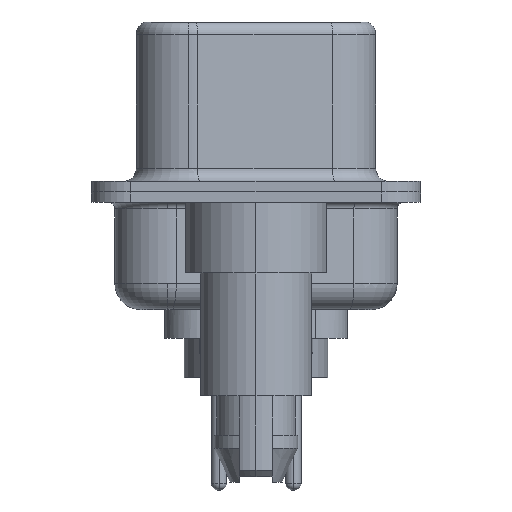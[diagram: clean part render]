
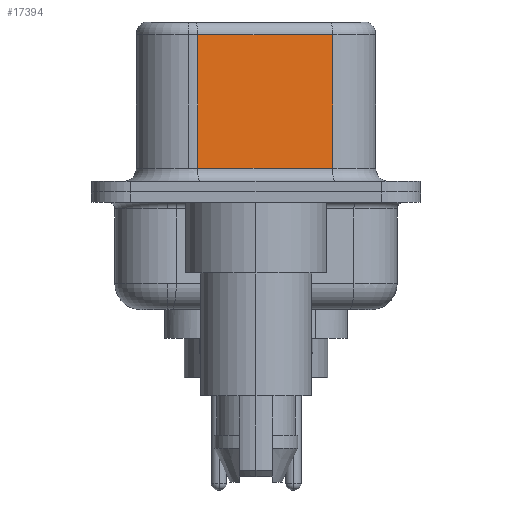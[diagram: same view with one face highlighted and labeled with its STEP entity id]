
A CAD part, left-side view. The second image highlights one B-rep face of the part: STEP entity #17394.
In plain terms, the highlighted planar face has unit normal (-0.985, -0.174, 0).
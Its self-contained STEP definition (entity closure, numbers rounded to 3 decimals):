
#341 = EDGE_CURVE ( 'NONE', #7643, #17818, #17907, .T. ) ;
#493 = EDGE_LOOP ( 'NONE', ( #12141, #4127, #10925, #8058 ) ) ;
#1292 = VERTEX_POINT ( 'NONE', #5120 ) ;
#1805 = CARTESIAN_POINT ( 'NONE',  ( 3.67, 2.233, 6.52 ) ) ;
#2773 = CARTESIAN_POINT ( 'NONE',  ( 4.58, -2.927, 0.9 ) ) ;
#2933 = VECTOR ( 'NONE', #13333, 1000. ) ;
#3874 = DIRECTION ( 'NONE',  ( 0.985, 0.174, 0. ) ) ;
#4127 = ORIENTED_EDGE ( 'NONE', *, *, #16135, .T. ) ;
#5120 = CARTESIAN_POINT ( 'NONE',  ( 4.58, -2.927, 6.02 ) ) ;
#5962 = VECTOR ( 'NONE', #15176, 1000. ) ;
#6122 = LINE ( 'NONE', #9501, #17211 ) ;
#7643 = VERTEX_POINT ( 'NONE', #9998 ) ;
#7668 = DIRECTION ( 'NONE',  ( 0.174, -0.985, 0. ) ) ;
#8058 = ORIENTED_EDGE ( 'NONE', *, *, #9245, .T. ) ;
#9245 = EDGE_CURVE ( 'NONE', #17818, #10702, #14181, .T. ) ;
#9501 = CARTESIAN_POINT ( 'NONE',  ( 4.58, -2.927, 6.52 ) ) ;
#9619 = PLANE ( 'NONE',  #16470 ) ;
#9998 = CARTESIAN_POINT ( 'NONE',  ( 3.67, 2.233, 6.02 ) ) ;
#10250 = LINE ( 'NONE', #17977, #5962 ) ;
#10702 = VERTEX_POINT ( 'NONE', #2773 ) ;
#10704 = VECTOR ( 'NONE', #7668, 1000. ) ;
#10925 = ORIENTED_EDGE ( 'NONE', *, *, #341, .T. ) ;
#11237 = EDGE_CURVE ( 'NONE', #1292, #10702, #6122, .T. ) ;
#12141 = ORIENTED_EDGE ( 'NONE', *, *, #11237, .F. ) ;
#12255 = CARTESIAN_POINT ( 'NONE',  ( 3.67, 2.233, 0.9 ) ) ;
#12589 = CARTESIAN_POINT ( 'NONE',  ( 4.58, -2.927, 6.52 ) ) ;
#13333 = DIRECTION ( 'NONE',  ( 0., 0., -1. ) ) ;
#14100 = DIRECTION ( 'NONE',  ( -0.174, 0.985, 0. ) ) ;
#14181 = LINE ( 'NONE', #17807, #10704 ) ;
#15176 = DIRECTION ( 'NONE',  ( -0.174, 0.985, 0. ) ) ;
#16135 = EDGE_CURVE ( 'NONE', #1292, #7643, #10250, .T. ) ;
#16470 = AXIS2_PLACEMENT_3D ( 'NONE', #12589, #3874, #14100 ) ;
#17211 = VECTOR ( 'NONE', #18190, 1000. ) ;
#17394 = ADVANCED_FACE ( 'NONE', ( #18144 ), #9619, .F. ) ;
#17807 = CARTESIAN_POINT ( 'NONE',  ( 4.58, -2.927, 0.9 ) ) ;
#17818 = VERTEX_POINT ( 'NONE', #12255 ) ;
#17907 = LINE ( 'NONE', #1805, #2933 ) ;
#17977 = CARTESIAN_POINT ( 'NONE',  ( 4.58, -2.927, 6.02 ) ) ;
#18144 = FACE_OUTER_BOUND ( 'NONE', #493, .T. ) ;
#18190 = DIRECTION ( 'NONE',  ( 0., 0., -1. ) ) ;
